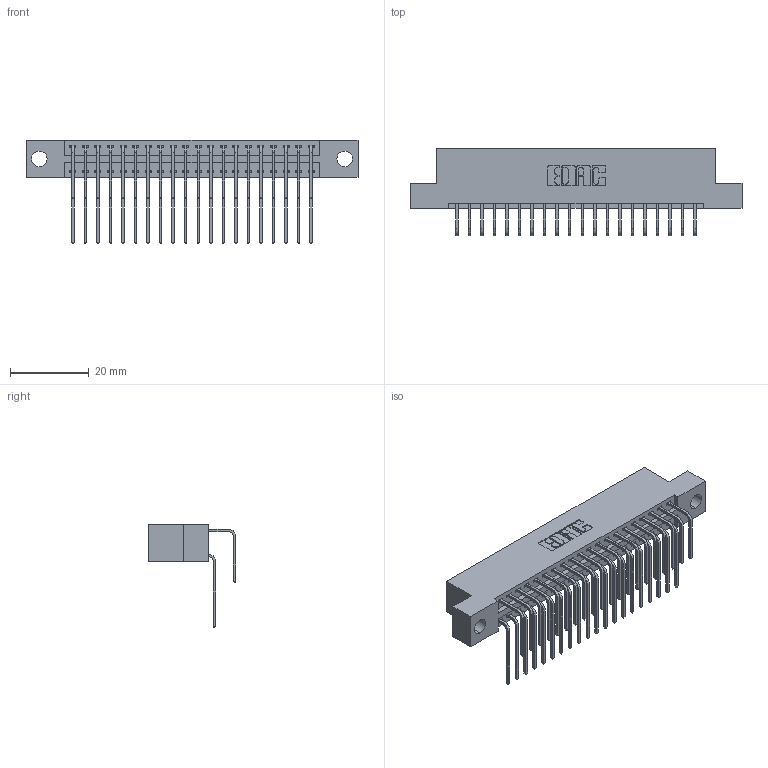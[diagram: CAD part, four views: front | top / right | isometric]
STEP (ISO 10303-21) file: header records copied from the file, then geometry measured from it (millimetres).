
FILE_DESCRIPTION (( 'STEP AP203' ), '1' );
FILE_NAME ('396-040-558-204.STEP', '2019-11-03T07:25:53', ( '' ), ( '' ), 'SwSTEP 2.0', 'SolidWorks 2016', '' );
FILE_SCHEMA (( 'CONFIG_CONTROL_DESIGN' ));
Length unit declared in the file: inch
Products named in the file (4): 396-040-558-204; 345-292-001_558 Tail - 2; 346 Part_Flush Mounting Lugs - 0.156 Dia-TH; 345-292-001_558 559 Tail - 1
Assembly tree (41 placements, depth 2):
  396-040-558-204
    346 Part_Flush Mounting Lugs - 0.156 Dia-TH
    345-292-001_558 559 Tail - 1  x20
    345-292-001_558 Tail - 2  x20
Bounding box: 84.07 x 22.16 x 26.16 mm (x, y, z)
Volume: 8170.3 mm3; surface area: 11805.2 mm2
Topology: 41 solids, 41 shells, 2282 faces, 6769 edges, 4458 vertices
Faces by surface type: plane 1556, cylinder 726
Entity records: 17801 total; most frequent: CARTESIAN_POINT 3015, ORIENTED_EDGE 2898, DIRECTION 2681, EDGE_CURVE 1449, LINE 1197, VECTOR 1197, VERTEX_POINT 962, AXIS2_PLACEMENT_3D 742
